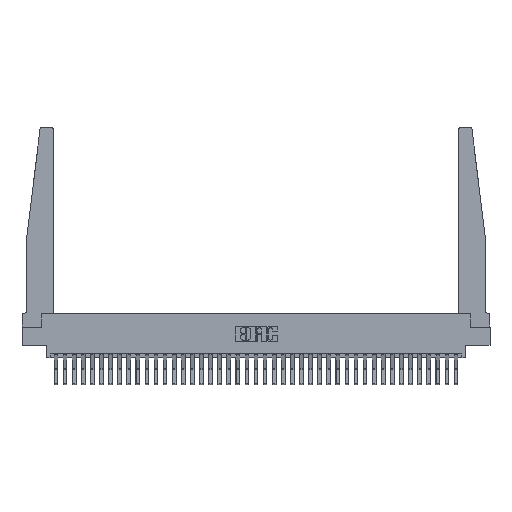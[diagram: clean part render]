
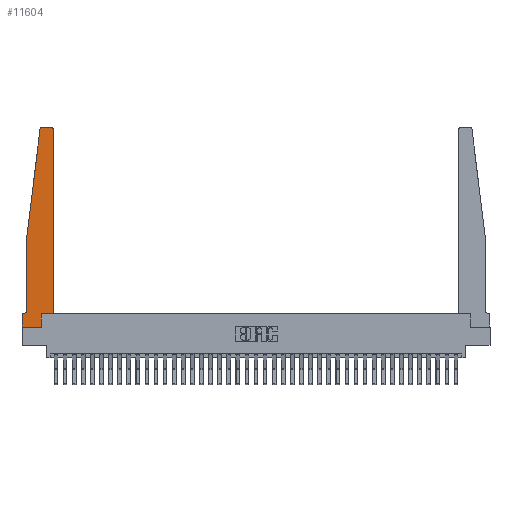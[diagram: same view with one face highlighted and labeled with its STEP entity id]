
A CAD part, top view. The second image highlights one B-rep face of the part: STEP entity #11604.
In plain terms, the highlighted planar face has unit normal (0, 0, 1).
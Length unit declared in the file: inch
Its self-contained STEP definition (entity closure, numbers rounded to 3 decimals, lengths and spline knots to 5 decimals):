
#423 = AXIS2_PLACEMENT_3D ( 'NONE', #18625, #2903, #21253 ) ;
#773 = DIRECTION ( 'NONE',  ( 0., 0., 1. ) ) ;
#1408 = EDGE_CURVE ( 'NONE', #32817, #18171, #7617, .T. ) ;
#1420 = ORIENTED_EDGE ( 'NONE', *, *, #16755, .T. ) ;
#1692 = LINE ( 'NONE', #14640, #14861 ) ;
#2511 = ORIENTED_EDGE ( 'NONE', *, *, #9082, .T. ) ;
#2590 = CARTESIAN_POINT ( 'NONE',  ( 0.27653, 2.75, 0.37 ) ) ;
#2903 = DIRECTION ( 'NONE',  ( 0., 0., -1. ) ) ;
#2962 = CARTESIAN_POINT ( 'NONE',  ( 0.27653, 2.72, 0.37 ) ) ;
#3343 = PLANE ( 'NONE',  #22575 ) ;
#3886 = EDGE_CURVE ( 'NONE', #30290, #32133, #7462, .T. ) ;
#4076 = ORIENTED_EDGE ( 'NONE', *, *, #17708, .T. ) ;
#4247 = CARTESIAN_POINT ( 'NONE',  ( 0., 0., 0.37 ) ) ;
#4334 = VECTOR ( 'NONE', #7424, 39.37008 ) ;
#4801 = DIRECTION ( 'NONE',  ( 0., 1., 0. ) ) ;
#5259 = CARTESIAN_POINT ( 'NONE',  ( 0.2605, 0., 0.37 ) ) ;
#5297 = VERTEX_POINT ( 'NONE', #19607 ) ;
#5621 = DIRECTION ( 'NONE',  ( 1., 0., 0. ) ) ;
#6048 = FACE_OUTER_BOUND ( 'NONE', #13026, .T. ) ;
#6119 = CARTESIAN_POINT ( 'NONE',  ( 0.395, 2.72, 0.37 ) ) ;
#6310 = CARTESIAN_POINT ( 'NONE',  ( 0.2605, 0.18, 0.37 ) ) ;
#6650 = LINE ( 'NONE', #33851, #26727 ) ;
#6705 = EDGE_CURVE ( 'NONE', #15605, #16517, #17454, .T. ) ;
#7424 = DIRECTION ( 'NONE',  ( 1., 0., 0. ) ) ;
#7446 = VECTOR ( 'NONE', #25866, 39.37008 ) ;
#7462 = CIRCLE ( 'NONE', #13665, 0.03 ) ;
#7511 = LINE ( 'NONE', #12533, #27558 ) ;
#7578 = CIRCLE ( 'NONE', #423, 0.05 ) ;
#7617 = LINE ( 'NONE', #29804, #27660 ) ;
#8754 = DIRECTION ( 'NONE',  ( 1., 0., 0. ) ) ;
#9082 = EDGE_CURVE ( 'NONE', #11363, #12129, #1692, .T. ) ;
#9587 = VERTEX_POINT ( 'NONE', #33783 ) ;
#10450 = ORIENTED_EDGE ( 'NONE', *, *, #13552, .T. ) ;
#11121 = EDGE_CURVE ( 'NONE', #30917, #9587, #11448, .T. ) ;
#11182 = CARTESIAN_POINT ( 'NONE',  ( 0., 0.1875, 0.37 ) ) ;
#11363 = VERTEX_POINT ( 'NONE', #12913 ) ;
#11448 = CIRCLE ( 'NONE', #32606, 0.03 ) ;
#11604 = ADVANCED_FACE ( 'NONE', ( #6048 ), #3343, .T. ) ;
#12129 = VERTEX_POINT ( 'NONE', #5259 ) ;
#12454 = VECTOR ( 'NONE', #30467, 39.37008 ) ;
#12533 = CARTESIAN_POINT ( 'NONE',  ( 0.425, 0.18, 0.37 ) ) ;
#12833 = EDGE_CURVE ( 'NONE', #32133, #32817, #16035, .T. ) ;
#12913 = CARTESIAN_POINT ( 'NONE',  ( 0., 0., 0.37 ) ) ;
#12977 = ORIENTED_EDGE ( 'NONE', *, *, #25842, .T. ) ;
#13026 = EDGE_LOOP ( 'NONE', ( #12977, #20477, #23156, #29143, #1420, #10450, #22866, #2511, #13967, #31475, #4076, #16210 ) ) ;
#13143 = LINE ( 'NONE', #18167, #33158 ) ;
#13552 = EDGE_CURVE ( 'NONE', #29314, #5297, #13143, .T. ) ;
#13665 = AXIS2_PLACEMENT_3D ( 'NONE', #2962, #21315, #5621 ) ;
#13967 = ORIENTED_EDGE ( 'NONE', *, *, #24186, .T. ) ;
#14169 = DIRECTION ( 'NONE',  ( 0., -1., 0. ) ) ;
#14640 = CARTESIAN_POINT ( 'NONE',  ( 0., 0., 0.37 ) ) ;
#14861 = VECTOR ( 'NONE', #17350, 39.37008 ) ;
#15605 = VERTEX_POINT ( 'NONE', #6310 ) ;
#16035 = LINE ( 'NONE', #23241, #7446 ) ;
#16210 = ORIENTED_EDGE ( 'NONE', *, *, #11121, .T. ) ;
#16517 = VERTEX_POINT ( 'NONE', #25610 ) ;
#16755 = EDGE_CURVE ( 'NONE', #18171, #29314, #7578, .T. ) ;
#17350 = DIRECTION ( 'NONE',  ( 1., 0., 0. ) ) ;
#17454 = LINE ( 'NONE', #17841, #4334 ) ;
#17708 = EDGE_CURVE ( 'NONE', #16517, #30917, #7511, .T. ) ;
#17841 = CARTESIAN_POINT ( 'NONE',  ( 0.425, 0.18, 0.37 ) ) ;
#17997 = VECTOR ( 'NONE', #24482, 39.37008 ) ;
#18167 = CARTESIAN_POINT ( 'NONE',  ( 0.065, 0.1875, 0.37 ) ) ;
#18171 = VERTEX_POINT ( 'NONE', #27267 ) ;
#18287 = CARTESIAN_POINT ( 'NONE',  ( 0.065, 1.25, 0.37 ) ) ;
#18625 = CARTESIAN_POINT ( 'NONE',  ( 0.015, 0.2375, 0.37 ) ) ;
#19154 = DIRECTION ( 'NONE',  ( 1., 0., 0. ) ) ;
#19375 = LINE ( 'NONE', #4247, #12454 ) ;
#19607 = CARTESIAN_POINT ( 'NONE',  ( 0., 0.1875, 0.37 ) ) ;
#20477 = ORIENTED_EDGE ( 'NONE', *, *, #3886, .T. ) ;
#21253 = DIRECTION ( 'NONE',  ( -1., 0., 0. ) ) ;
#21315 = DIRECTION ( 'NONE',  ( 0., 0., 1. ) ) ;
#22575 = AXIS2_PLACEMENT_3D ( 'NONE', #11182, #773, #19154 ) ;
#22866 = ORIENTED_EDGE ( 'NONE', *, *, #25641, .T. ) ;
#23156 = ORIENTED_EDGE ( 'NONE', *, *, #12833, .T. ) ;
#23241 = CARTESIAN_POINT ( 'NONE',  ( 0.065, 1.25, 0.37 ) ) ;
#24186 = EDGE_CURVE ( 'NONE', #12129, #15605, #31892, .T. ) ;
#24456 = DIRECTION ( 'NONE',  ( 0., 0., 1. ) ) ;
#24482 = DIRECTION ( 'NONE',  ( 0., 1., 0. ) ) ;
#25610 = CARTESIAN_POINT ( 'NONE',  ( 0.425, 0.18, 0.37 ) ) ;
#25641 = EDGE_CURVE ( 'NONE', #5297, #11363, #19375, .T. ) ;
#25842 = EDGE_CURVE ( 'NONE', #9587, #30290, #6650, .T. ) ;
#25866 = DIRECTION ( 'NONE',  ( -0.122, -0.992, 0. ) ) ;
#26727 = VECTOR ( 'NONE', #28603, 39.37008 ) ;
#27267 = CARTESIAN_POINT ( 'NONE',  ( 0.065, 0.2375, 0.37 ) ) ;
#27558 = VECTOR ( 'NONE', #4801, 39.37008 ) ;
#27660 = VECTOR ( 'NONE', #14169, 39.37008 ) ;
#28603 = DIRECTION ( 'NONE',  ( -1., 0., 0. ) ) ;
#28668 = DIRECTION ( 'NONE',  ( -1., 0., 0. ) ) ;
#29143 = ORIENTED_EDGE ( 'NONE', *, *, #1408, .T. ) ;
#29314 = VERTEX_POINT ( 'NONE', #29351 ) ;
#29351 = CARTESIAN_POINT ( 'NONE',  ( 0.015, 0.1875, 0.37 ) ) ;
#29804 = CARTESIAN_POINT ( 'NONE',  ( 0.065, 1.25, 0.37 ) ) ;
#30290 = VERTEX_POINT ( 'NONE', #2590 ) ;
#30467 = DIRECTION ( 'NONE',  ( 0., -1., 0. ) ) ;
#30917 = VERTEX_POINT ( 'NONE', #33798 ) ;
#31475 = ORIENTED_EDGE ( 'NONE', *, *, #6705, .T. ) ;
#31892 = LINE ( 'NONE', #32361, #17997 ) ;
#32133 = VERTEX_POINT ( 'NONE', #33503 ) ;
#32361 = CARTESIAN_POINT ( 'NONE',  ( 0.2605, 0.18, 0.37 ) ) ;
#32606 = AXIS2_PLACEMENT_3D ( 'NONE', #6119, #24456, #8754 ) ;
#32817 = VERTEX_POINT ( 'NONE', #18287 ) ;
#33158 = VECTOR ( 'NONE', #28668, 39.37008 ) ;
#33503 = CARTESIAN_POINT ( 'NONE',  ( 0.24675, 2.72367, 0.37 ) ) ;
#33783 = CARTESIAN_POINT ( 'NONE',  ( 0.395, 2.75, 0.37 ) ) ;
#33798 = CARTESIAN_POINT ( 'NONE',  ( 0.425, 2.72, 0.37 ) ) ;
#33851 = CARTESIAN_POINT ( 'NONE',  ( 0.25, 2.75, 0.37 ) ) ;
